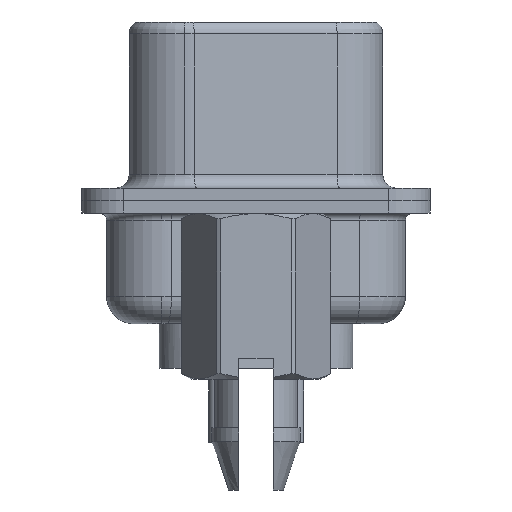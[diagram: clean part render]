
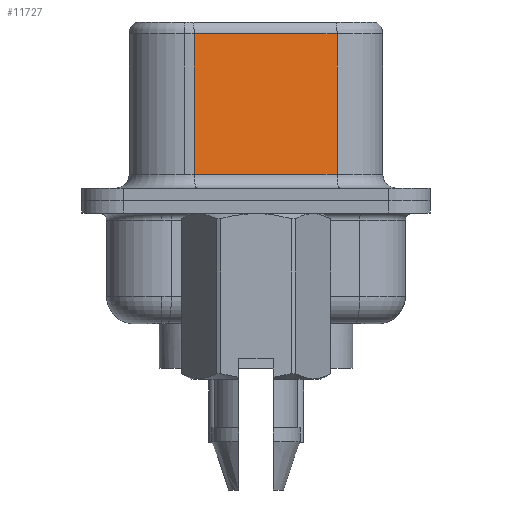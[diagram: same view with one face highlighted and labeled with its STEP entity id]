
A CAD part, left-side view. The second image highlights one B-rep face of the part: STEP entity #11727.
In plain terms, the highlighted planar face has unit normal (-0.985, -0.174, 0).
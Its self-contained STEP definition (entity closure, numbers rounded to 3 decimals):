
#340 = EDGE_CURVE ( 'NONE', #16056, #9135, #1395, .T. ) ;
#589 = DIRECTION ( 'NONE',  ( 0., 0., -1. ) ) ;
#644 = DIRECTION ( 'NONE',  ( 0.174, -0.985, 0. ) ) ;
#1071 = CARTESIAN_POINT ( 'NONE',  ( 4.575, -2.927, 0.95 ) ) ;
#1395 = LINE ( 'NONE', #1071, #18848 ) ;
#1495 = LINE ( 'NONE', #8717, #8929 ) ;
#1592 = DIRECTION ( 'NONE',  ( -0.174, 0.985, 0. ) ) ;
#1720 = ORIENTED_EDGE ( 'NONE', *, *, #340, .T. ) ;
#2077 = CARTESIAN_POINT ( 'NONE',  ( 4.575, -2.927, 6.02 ) ) ;
#2250 = LINE ( 'NONE', #5998, #8151 ) ;
#4532 = VERTEX_POINT ( 'NONE', #2077 ) ;
#5293 = FACE_OUTER_BOUND ( 'NONE', #7185, .T. ) ;
#5949 = DIRECTION ( 'NONE',  ( 0., 0., -1. ) ) ;
#5998 = CARTESIAN_POINT ( 'NONE',  ( 3.665, 2.233, 6.52 ) ) ;
#6496 = CARTESIAN_POINT ( 'NONE',  ( 3.665, 2.233, 0.95 ) ) ;
#7185 = EDGE_LOOP ( 'NONE', ( #12934, #18489, #7412, #1720 ) ) ;
#7412 = ORIENTED_EDGE ( 'NONE', *, *, #14796, .T. ) ;
#7495 = LINE ( 'NONE', #18030, #20646 ) ;
#8151 = VECTOR ( 'NONE', #589, 1000. ) ;
#8717 = CARTESIAN_POINT ( 'NONE',  ( 4.575, -2.927, 6.02 ) ) ;
#8929 = VECTOR ( 'NONE', #1592, 1000. ) ;
#9135 = VERTEX_POINT ( 'NONE', #17885 ) ;
#11257 = EDGE_CURVE ( 'NONE', #4532, #15710, #1495, .T. ) ;
#11727 = ADVANCED_FACE ( 'NONE', ( #5293 ), #16971, .F. ) ;
#11864 = DIRECTION ( 'NONE',  ( -0.174, 0.985, 0. ) ) ;
#12934 = ORIENTED_EDGE ( 'NONE', *, *, #18168, .F. ) ;
#14234 = CARTESIAN_POINT ( 'NONE',  ( 3.665, 2.233, 6.02 ) ) ;
#14796 = EDGE_CURVE ( 'NONE', #15710, #16056, #2250, .T. ) ;
#15710 = VERTEX_POINT ( 'NONE', #14234 ) ;
#16056 = VERTEX_POINT ( 'NONE', #6496 ) ;
#16908 = CARTESIAN_POINT ( 'NONE',  ( 4.575, -2.927, 6.52 ) ) ;
#16971 = PLANE ( 'NONE',  #18345 ) ;
#17885 = CARTESIAN_POINT ( 'NONE',  ( 4.575, -2.927, 0.95 ) ) ;
#18030 = CARTESIAN_POINT ( 'NONE',  ( 4.575, -2.927, 6.52 ) ) ;
#18168 = EDGE_CURVE ( 'NONE', #4532, #9135, #7495, .T. ) ;
#18345 = AXIS2_PLACEMENT_3D ( 'NONE', #16908, #22084, #11864 ) ;
#18489 = ORIENTED_EDGE ( 'NONE', *, *, #11257, .T. ) ;
#18848 = VECTOR ( 'NONE', #644, 1000. ) ;
#20646 = VECTOR ( 'NONE', #5949, 1000. ) ;
#22084 = DIRECTION ( 'NONE',  ( 0.985, 0.174, 0. ) ) ;
